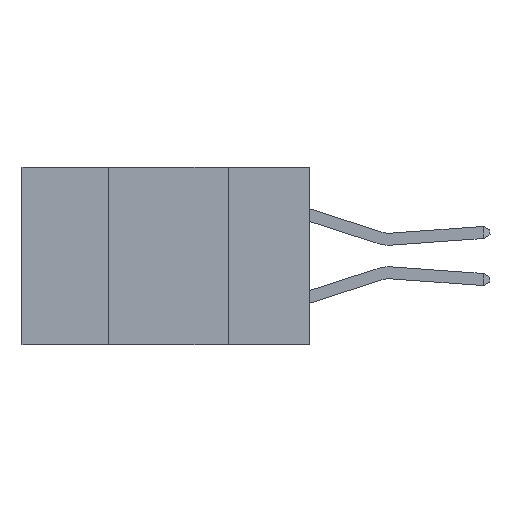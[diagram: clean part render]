
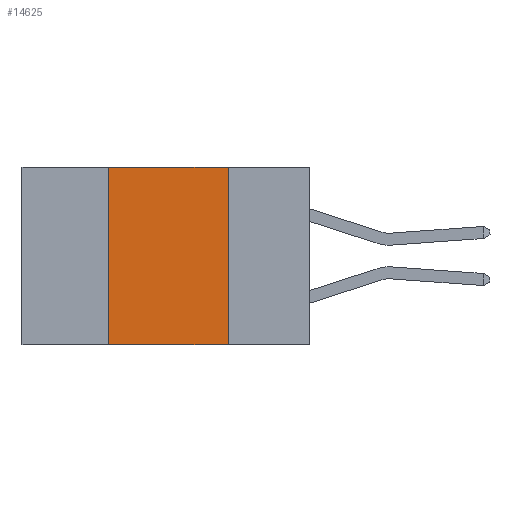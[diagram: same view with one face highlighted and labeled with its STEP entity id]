
A CAD part, left-side view. The second image highlights one B-rep face of the part: STEP entity #14625.
In plain terms, the highlighted planar face has unit normal (-1, 0, 0).
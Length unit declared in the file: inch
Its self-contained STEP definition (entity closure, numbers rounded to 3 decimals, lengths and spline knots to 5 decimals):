
#1120 = LINE ( 'NONE', #17006, #19740 ) ;
#3942 = EDGE_CURVE ( 'NONE', #10510, #14170, #1120, .T. ) ;
#4331 = DIRECTION ( 'NONE',  ( 0., -1., 0. ) ) ;
#4840 = PLANE ( 'NONE',  #24921 ) ;
#5909 = CARTESIAN_POINT ( 'NONE',  ( 0., 0.6, -0.37 ) ) ;
#6524 = EDGE_LOOP ( 'NONE', ( #11316, #11173, #9852, #15118 ) ) ;
#6574 = EDGE_CURVE ( 'NONE', #17978, #10510, #19487, .T. ) ;
#7577 = CARTESIAN_POINT ( 'NONE',  ( 0., 0.17, 0. ) ) ;
#8699 = CARTESIAN_POINT ( 'NONE',  ( 0., 0.42, -0.37 ) ) ;
#8779 = DIRECTION ( 'NONE',  ( 0., 0., -1. ) ) ;
#8962 = CARTESIAN_POINT ( 'NONE',  ( 0., 0.17, -0.37 ) ) ;
#9228 = DIRECTION ( 'NONE',  ( 0., -1., 0. ) ) ;
#9852 = ORIENTED_EDGE ( 'NONE', *, *, #6574, .F. ) ;
#10510 = VERTEX_POINT ( 'NONE', #17748 ) ;
#10651 = CARTESIAN_POINT ( 'NONE',  ( 0., 0.42, 0. ) ) ;
#11173 = ORIENTED_EDGE ( 'NONE', *, *, #3942, .F. ) ;
#11316 = ORIENTED_EDGE ( 'NONE', *, *, #23159, .F. ) ;
#11460 = VECTOR ( 'NONE', #16608, 39.37008 ) ;
#12009 = DIRECTION ( 'NONE',  ( 0., 0., -1. ) ) ;
#12948 = DIRECTION ( 'NONE',  ( 1., 0., 0. ) ) ;
#13171 = LINE ( 'NONE', #23912, #24572 ) ;
#14170 = VERTEX_POINT ( 'NONE', #7577 ) ;
#14625 = ADVANCED_FACE ( 'NONE', ( #19330 ), #4840, .F. ) ;
#15118 = ORIENTED_EDGE ( 'NONE', *, *, #18087, .T. ) ;
#16608 = DIRECTION ( 'NONE',  ( 0., 0., 1. ) ) ;
#17006 = CARTESIAN_POINT ( 'NONE',  ( 0., 0.6, 0. ) ) ;
#17203 = VERTEX_POINT ( 'NONE', #8962 ) ;
#17748 = CARTESIAN_POINT ( 'NONE',  ( 0., 0.42, 0. ) ) ;
#17978 = VERTEX_POINT ( 'NONE', #8699 ) ;
#18087 = EDGE_CURVE ( 'NONE', #17978, #17203, #23591, .T. ) ;
#18353 = VECTOR ( 'NONE', #4331, 39.37008 ) ;
#19330 = FACE_OUTER_BOUND ( 'NONE', #6524, .T. ) ;
#19487 = LINE ( 'NONE', #10651, #11460 ) ;
#19740 = VECTOR ( 'NONE', #9228, 39.37008 ) ;
#20584 = CARTESIAN_POINT ( 'NONE',  ( 0., 0.6, 0. ) ) ;
#23159 = EDGE_CURVE ( 'NONE', #14170, #17203, #13171, .T. ) ;
#23591 = LINE ( 'NONE', #5909, #18353 ) ;
#23912 = CARTESIAN_POINT ( 'NONE',  ( 0., 0.17, 0. ) ) ;
#24572 = VECTOR ( 'NONE', #12009, 39.37008 ) ;
#24921 = AXIS2_PLACEMENT_3D ( 'NONE', #20584, #12948, #8779 ) ;
